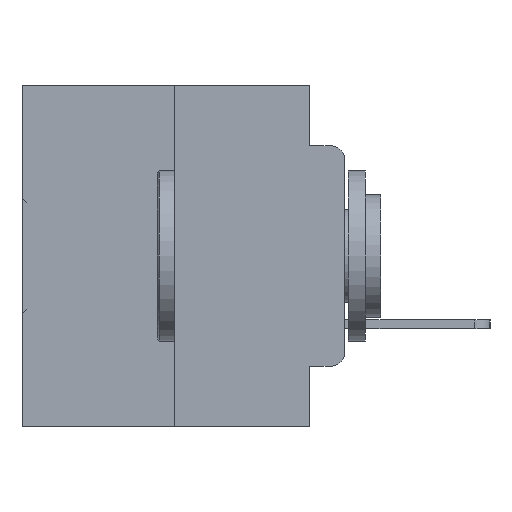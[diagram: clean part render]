
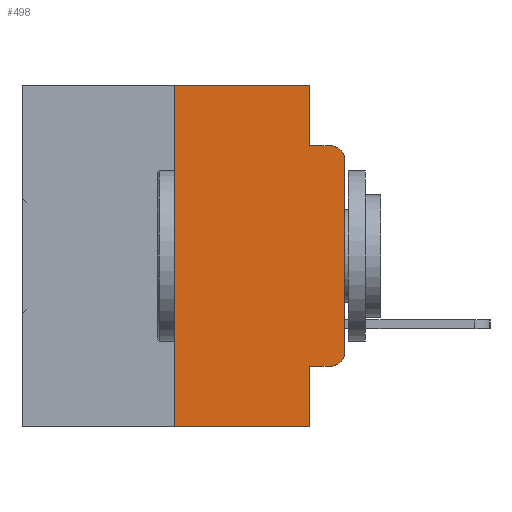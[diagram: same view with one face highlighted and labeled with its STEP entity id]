
A CAD part, left-side view. The second image highlights one B-rep face of the part: STEP entity #498.
In plain terms, the highlighted planar face has unit normal (-1, 0, 0).
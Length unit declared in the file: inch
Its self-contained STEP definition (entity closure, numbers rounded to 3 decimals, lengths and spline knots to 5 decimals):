
#92 = LINE ( 'NONE', #32841, #5734 ) ;
#373 = ORIENTED_EDGE ( 'NONE', *, *, #22202, .T. ) ;
#478 = LINE ( 'NONE', #5431, #7701 ) ;
#498 = ADVANCED_FACE ( 'NONE', ( #30008 ), #32104, .F. ) ;
#841 = ORIENTED_EDGE ( 'NONE', *, *, #33627, .F. ) ;
#892 = DIRECTION ( 'NONE',  ( 1., 0., 0. ) ) ;
#1279 = ORIENTED_EDGE ( 'NONE', *, *, #25002, .F. ) ;
#1772 = VERTEX_POINT ( 'NONE', #26472 ) ;
#2076 = EDGE_CURVE ( 'NONE', #11755, #4356, #92, .T. ) ;
#2191 = VECTOR ( 'NONE', #30727, 39.37008 ) ;
#2278 = CARTESIAN_POINT ( 'NONE',  ( 0., 0.02, -0.3915 ) ) ;
#3092 = CARTESIAN_POINT ( 'NONE',  ( 0., 0.473, -0.5 ) ) ;
#3125 = CARTESIAN_POINT ( 'NONE',  ( 0., 0.051, -0.0885 ) ) ;
#3696 = CARTESIAN_POINT ( 'NONE',  ( 0., 0.02, -0.4115 ) ) ;
#3931 = ORIENTED_EDGE ( 'NONE', *, *, #31901, .F. ) ;
#4356 = VERTEX_POINT ( 'NONE', #23518 ) ;
#5027 = DIRECTION ( 'NONE',  ( 0., 0., -1. ) ) ;
#5357 = CIRCLE ( 'NONE', #29637, 0.02 ) ;
#5431 = CARTESIAN_POINT ( 'NONE',  ( 0., 0.051, 0. ) ) ;
#5514 = VERTEX_POINT ( 'NONE', #22686 ) ;
#5734 = VECTOR ( 'NONE', #9718, 39.37008 ) ;
#5883 = VERTEX_POINT ( 'NONE', #3125 ) ;
#7074 = VECTOR ( 'NONE', #13530, 39.37008 ) ;
#7353 = DIRECTION ( 'NONE',  ( 0., -1., 0. ) ) ;
#7701 = VECTOR ( 'NONE', #23404, 39.37008 ) ;
#8031 = ORIENTED_EDGE ( 'NONE', *, *, #16882, .T. ) ;
#8609 = DIRECTION ( 'NONE',  ( -1., 0., 0. ) ) ;
#8667 = AXIS2_PLACEMENT_3D ( 'NONE', #11489, #892, #19318 ) ;
#8792 = VERTEX_POINT ( 'NONE', #3696 ) ;
#9586 = VERTEX_POINT ( 'NONE', #15145 ) ;
#9718 = DIRECTION ( 'NONE',  ( 0., -1., 0. ) ) ;
#9965 = CARTESIAN_POINT ( 'NONE',  ( 0., 0.051, -0.4115 ) ) ;
#10890 = EDGE_LOOP ( 'NONE', ( #27407, #373, #1279, #29828, #17026, #3931, #26208, #841, #8031, #29432 ) ) ;
#11489 = CARTESIAN_POINT ( 'NONE',  ( 0., 0.473, 0. ) ) ;
#11755 = VERTEX_POINT ( 'NONE', #29794 ) ;
#13038 = LINE ( 'NONE', #16194, #33557 ) ;
#13136 = VECTOR ( 'NONE', #18159, 39.37008 ) ;
#13530 = DIRECTION ( 'NONE',  ( 0., 0., -1. ) ) ;
#14072 = LINE ( 'NONE', #26420, #7074 ) ;
#15145 = CARTESIAN_POINT ( 'NONE',  ( 0., 0.051, -0.4115 ) ) ;
#15792 = CARTESIAN_POINT ( 'NONE',  ( 0., 0.051, -0.5 ) ) ;
#15895 = LINE ( 'NONE', #9965, #21846 ) ;
#16194 = CARTESIAN_POINT ( 'NONE',  ( 0., 0., 0. ) ) ;
#16311 = VERTEX_POINT ( 'NONE', #18101 ) ;
#16882 = EDGE_CURVE ( 'NONE', #9586, #8792, #15895, .T. ) ;
#17026 = ORIENTED_EDGE ( 'NONE', *, *, #2076, .F. ) ;
#17963 = CARTESIAN_POINT ( 'NONE',  ( 0., 0.02, -0.0885 ) ) ;
#17983 = VERTEX_POINT ( 'NONE', #15792 ) ;
#18101 = CARTESIAN_POINT ( 'NONE',  ( 0., 0.25, -0.5 ) ) ;
#18159 = DIRECTION ( 'NONE',  ( 0., 0., 1. ) ) ;
#19318 = DIRECTION ( 'NONE',  ( 0., 0., -1. ) ) ;
#19978 = LINE ( 'NONE', #28352, #13136 ) ;
#20551 = DIRECTION ( 'NONE',  ( -1., 0., 0. ) ) ;
#21846 = VECTOR ( 'NONE', #7353, 39.37008 ) ;
#22202 = EDGE_CURVE ( 'NONE', #1772, #31828, #33669, .T. ) ;
#22686 = CARTESIAN_POINT ( 'NONE',  ( 0., 0., -0.3915 ) ) ;
#23404 = DIRECTION ( 'NONE',  ( 0., 0., -1. ) ) ;
#23518 = CARTESIAN_POINT ( 'NONE',  ( 0., 0.051, 0. ) ) ;
#23652 = DIRECTION ( 'NONE',  ( 0., 0., 1. ) ) ;
#23879 = DIRECTION ( 'NONE',  ( 0., -1., 0. ) ) ;
#23932 = EDGE_CURVE ( 'NONE', #5514, #1772, #13038, .T. ) ;
#24086 = CARTESIAN_POINT ( 'NONE',  ( 0., 0.02, -0.1085 ) ) ;
#25002 = EDGE_CURVE ( 'NONE', #5883, #31828, #29035, .T. ) ;
#25159 = AXIS2_PLACEMENT_3D ( 'NONE', #24086, #8609, #26684 ) ;
#25541 = CARTESIAN_POINT ( 'NONE',  ( 0., 0.051, -0.0885 ) ) ;
#26208 = ORIENTED_EDGE ( 'NONE', *, *, #26233, .T. ) ;
#26233 = EDGE_CURVE ( 'NONE', #16311, #17983, #29349, .T. ) ;
#26420 = CARTESIAN_POINT ( 'NONE',  ( 0., 0.051, 0. ) ) ;
#26472 = CARTESIAN_POINT ( 'NONE',  ( 0., 0., -0.1085 ) ) ;
#26684 = DIRECTION ( 'NONE',  ( 0., 0., -1. ) ) ;
#26725 = EDGE_CURVE ( 'NONE', #4356, #5883, #14072, .T. ) ;
#27407 = ORIENTED_EDGE ( 'NONE', *, *, #23932, .T. ) ;
#28352 = CARTESIAN_POINT ( 'NONE',  ( 0., 0.25, 0. ) ) ;
#28553 = VECTOR ( 'NONE', #23879, 39.37008 ) ;
#29035 = LINE ( 'NONE', #25541, #2191 ) ;
#29349 = LINE ( 'NONE', #3092, #28553 ) ;
#29432 = ORIENTED_EDGE ( 'NONE', *, *, #30618, .T. ) ;
#29637 = AXIS2_PLACEMENT_3D ( 'NONE', #2278, #20551, #5027 ) ;
#29794 = CARTESIAN_POINT ( 'NONE',  ( 0., 0.25, 0. ) ) ;
#29828 = ORIENTED_EDGE ( 'NONE', *, *, #26725, .F. ) ;
#30008 = FACE_OUTER_BOUND ( 'NONE', #10890, .T. ) ;
#30618 = EDGE_CURVE ( 'NONE', #8792, #5514, #5357, .T. ) ;
#30727 = DIRECTION ( 'NONE',  ( 0., -1., 0. ) ) ;
#31828 = VERTEX_POINT ( 'NONE', #17963 ) ;
#31901 = EDGE_CURVE ( 'NONE', #16311, #11755, #19978, .T. ) ;
#32104 = PLANE ( 'NONE',  #8667 ) ;
#32841 = CARTESIAN_POINT ( 'NONE',  ( 0., 0.473, 0. ) ) ;
#33557 = VECTOR ( 'NONE', #23652, 39.37008 ) ;
#33627 = EDGE_CURVE ( 'NONE', #9586, #17983, #478, .T. ) ;
#33669 = CIRCLE ( 'NONE', #25159, 0.02 ) ;
